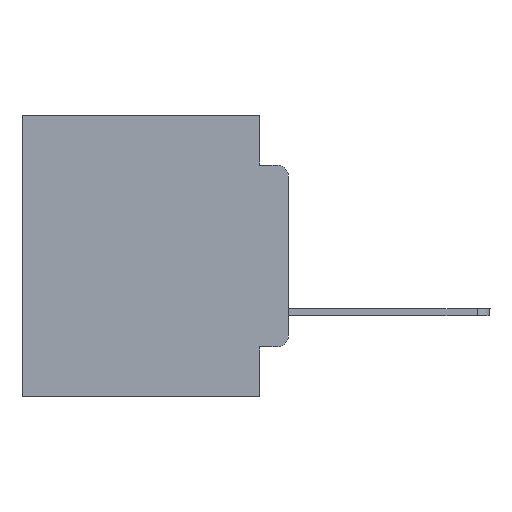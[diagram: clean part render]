
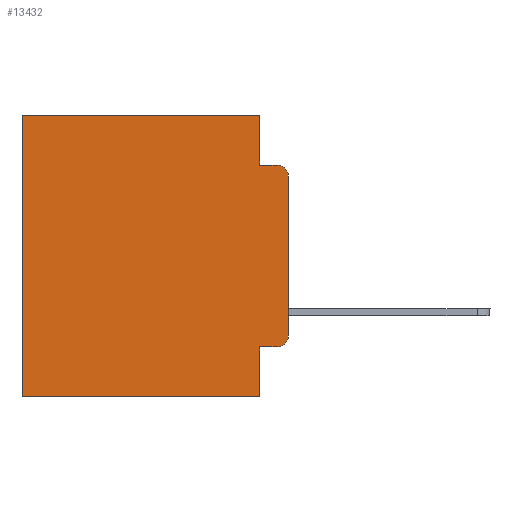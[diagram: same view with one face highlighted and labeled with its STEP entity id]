
A CAD part, left-side view. The second image highlights one B-rep face of the part: STEP entity #13432.
In plain terms, the highlighted planar face has unit normal (-1, 0, 0).
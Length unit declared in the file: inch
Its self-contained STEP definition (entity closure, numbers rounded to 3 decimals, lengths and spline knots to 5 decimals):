
#518 = ORIENTED_EDGE ( 'NONE', *, *, #16250, .T. ) ;
#1212 = DIRECTION ( 'NONE',  ( 0., 0., -1. ) ) ;
#1263 = EDGE_CURVE ( 'NONE', #12335, #18443, #17397, .T. ) ;
#1627 = CARTESIAN_POINT ( 'NONE',  ( 0.298, 0., 0. ) ) ;
#2224 = LINE ( 'NONE', #15815, #9255 ) ;
#2636 = CARTESIAN_POINT ( 'NONE',  ( 0.298, 0., -0.3915 ) ) ;
#2900 = ORIENTED_EDGE ( 'NONE', *, *, #4360, .T. ) ;
#3095 = VERTEX_POINT ( 'NONE', #9264 ) ;
#3267 = CARTESIAN_POINT ( 'NONE',  ( 0.298, 0.02, -0.1085 ) ) ;
#3769 = CARTESIAN_POINT ( 'NONE',  ( 0.298, 0.02, -0.3915 ) ) ;
#3894 = CARTESIAN_POINT ( 'NONE',  ( 0.298, 0., 0. ) ) ;
#4077 = CARTESIAN_POINT ( 'NONE',  ( 0.298, 0.473, -0.5 ) ) ;
#4360 = EDGE_CURVE ( 'NONE', #9191, #13442, #15266, .T. ) ;
#5292 = ORIENTED_EDGE ( 'NONE', *, *, #14973, .F. ) ;
#5374 = VERTEX_POINT ( 'NONE', #4077 ) ;
#5416 = DIRECTION ( 'NONE',  ( 1., 0., 0. ) ) ;
#5613 = VECTOR ( 'NONE', #16143, 39.37008 ) ;
#5790 = LINE ( 'NONE', #3894, #23610 ) ;
#6207 = LINE ( 'NONE', #7759, #9163 ) ;
#7439 = EDGE_CURVE ( 'NONE', #12383, #13442, #13682, .T. ) ;
#7759 = CARTESIAN_POINT ( 'NONE',  ( 0.298, 0.473, 0. ) ) ;
#7944 = ORIENTED_EDGE ( 'NONE', *, *, #7439, .F. ) ;
#8008 = VERTEX_POINT ( 'NONE', #2636 ) ;
#8152 = CARTESIAN_POINT ( 'NONE',  ( 0.298, 0.051, 0. ) ) ;
#9163 = VECTOR ( 'NONE', #23341, 39.37008 ) ;
#9191 = VERTEX_POINT ( 'NONE', #15581 ) ;
#9255 = VECTOR ( 'NONE', #10291, 39.37008 ) ;
#9264 = CARTESIAN_POINT ( 'NONE',  ( 0.298, 0.473, 0. ) ) ;
#9314 = CARTESIAN_POINT ( 'NONE',  ( 0.298, 0.051, 0. ) ) ;
#9318 = ORIENTED_EDGE ( 'NONE', *, *, #19044, .F. ) ;
#9898 = DIRECTION ( 'NONE',  ( 0., 0., -1. ) ) ;
#10291 = DIRECTION ( 'NONE',  ( 0., 1., 0. ) ) ;
#10637 = CARTESIAN_POINT ( 'NONE',  ( 0.298, 0.051, -0.4115 ) ) ;
#10774 = AXIS2_PLACEMENT_3D ( 'NONE', #3267, #15051, #22918 ) ;
#10837 = CARTESIAN_POINT ( 'NONE',  ( 0.298, 0.051, 0. ) ) ;
#10866 = ORIENTED_EDGE ( 'NONE', *, *, #20336, .T. ) ;
#11074 = PLANE ( 'NONE',  #16168 ) ;
#11203 = CARTESIAN_POINT ( 'NONE',  ( 0.298, 0., 0. ) ) ;
#12234 = ORIENTED_EDGE ( 'NONE', *, *, #13061, .T. ) ;
#12335 = VERTEX_POINT ( 'NONE', #10637 ) ;
#12383 = VERTEX_POINT ( 'NONE', #24185 ) ;
#13061 = EDGE_CURVE ( 'NONE', #3095, #5374, #6207, .T. ) ;
#13432 = ADVANCED_FACE ( 'NONE', ( #23045 ), #11074, .F. ) ;
#13442 = VERTEX_POINT ( 'NONE', #19173 ) ;
#13682 = LINE ( 'NONE', #19868, #21638 ) ;
#14132 = CARTESIAN_POINT ( 'NONE',  ( 0.298, 0.02, -0.4115 ) ) ;
#14580 = VERTEX_POINT ( 'NONE', #8152 ) ;
#14973 = EDGE_CURVE ( 'NONE', #9191, #8008, #5790, .T. ) ;
#15051 = DIRECTION ( 'NONE',  ( -1., 0., 0. ) ) ;
#15266 = CIRCLE ( 'NONE', #10774, 0.02 ) ;
#15537 = EDGE_LOOP ( 'NONE', ( #5292, #2900, #7944, #9318, #25201, #12234, #24126, #23078, #10866, #518 ) ) ;
#15581 = CARTESIAN_POINT ( 'NONE',  ( 0.298, 0., -0.1085 ) ) ;
#15673 = VECTOR ( 'NONE', #1212, 39.37008 ) ;
#15815 = CARTESIAN_POINT ( 'NONE',  ( 0.298, 0., -0.5 ) ) ;
#16143 = DIRECTION ( 'NONE',  ( 0., -1., 0. ) ) ;
#16168 = AXIS2_PLACEMENT_3D ( 'NONE', #11203, #5416, #19050 ) ;
#16250 = EDGE_CURVE ( 'NONE', #22601, #8008, #23244, .T. ) ;
#16330 = EDGE_CURVE ( 'NONE', #18443, #5374, #2224, .T. ) ;
#17131 = VECTOR ( 'NONE', #21019, 39.37008 ) ;
#17397 = LINE ( 'NONE', #9314, #24348 ) ;
#17621 = DIRECTION ( 'NONE',  ( -1., 0., 0. ) ) ;
#18443 = VERTEX_POINT ( 'NONE', #24288 ) ;
#18845 = LINE ( 'NONE', #1627, #17131 ) ;
#19044 = EDGE_CURVE ( 'NONE', #14580, #12383, #20871, .T. ) ;
#19050 = DIRECTION ( 'NONE',  ( 0., 0., -1. ) ) ;
#19173 = CARTESIAN_POINT ( 'NONE',  ( 0.298, 0.02, -0.0885 ) ) ;
#19868 = CARTESIAN_POINT ( 'NONE',  ( 0.298, 0.051, -0.0885 ) ) ;
#19944 = AXIS2_PLACEMENT_3D ( 'NONE', #3769, #17621, #21882 ) ;
#20336 = EDGE_CURVE ( 'NONE', #12335, #22601, #24045, .T. ) ;
#20505 = EDGE_CURVE ( 'NONE', #14580, #3095, #18845, .T. ) ;
#20871 = LINE ( 'NONE', #10837, #15673 ) ;
#21019 = DIRECTION ( 'NONE',  ( 0., 1., 0. ) ) ;
#21548 = DIRECTION ( 'NONE',  ( 0., -1., 0. ) ) ;
#21638 = VECTOR ( 'NONE', #21548, 39.37008 ) ;
#21882 = DIRECTION ( 'NONE',  ( 0., 0., -1. ) ) ;
#22601 = VERTEX_POINT ( 'NONE', #14132 ) ;
#22918 = DIRECTION ( 'NONE',  ( 0., 0., -1. ) ) ;
#23045 = FACE_OUTER_BOUND ( 'NONE', #15537, .T. ) ;
#23078 = ORIENTED_EDGE ( 'NONE', *, *, #1263, .F. ) ;
#23244 = CIRCLE ( 'NONE', #19944, 0.02 ) ;
#23341 = DIRECTION ( 'NONE',  ( 0., 0., -1. ) ) ;
#23610 = VECTOR ( 'NONE', #9898, 39.37008 ) ;
#24045 = LINE ( 'NONE', #24287, #5613 ) ;
#24126 = ORIENTED_EDGE ( 'NONE', *, *, #16330, .F. ) ;
#24185 = CARTESIAN_POINT ( 'NONE',  ( 0.298, 0.051, -0.0885 ) ) ;
#24287 = CARTESIAN_POINT ( 'NONE',  ( 0.298, 0.051, -0.4115 ) ) ;
#24288 = CARTESIAN_POINT ( 'NONE',  ( 0.298, 0.051, -0.5 ) ) ;
#24348 = VECTOR ( 'NONE', #25025, 39.37008 ) ;
#25025 = DIRECTION ( 'NONE',  ( 0., 0., -1. ) ) ;
#25201 = ORIENTED_EDGE ( 'NONE', *, *, #20505, .T. ) ;
